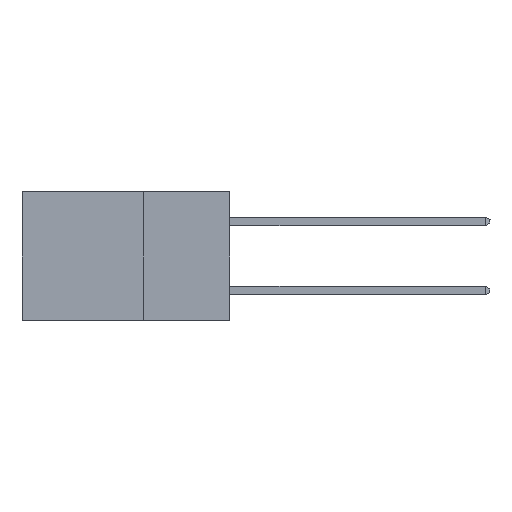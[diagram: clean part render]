
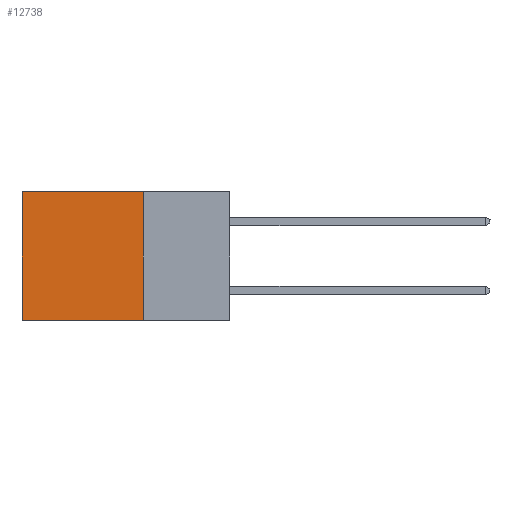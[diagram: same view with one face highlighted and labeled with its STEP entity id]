
A CAD part, left-side view. The second image highlights one B-rep face of the part: STEP entity #12738.
In plain terms, the highlighted planar face has unit normal (-1, 0, 0).
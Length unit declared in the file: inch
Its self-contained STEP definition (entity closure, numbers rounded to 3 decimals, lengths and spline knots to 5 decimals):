
#794 = CARTESIAN_POINT ( 'NONE',  ( 0.2615, 0.25, -0.37 ) ) ;
#1117 = LINE ( 'NONE', #12766, #20195 ) ;
#1715 = DIRECTION ( 'NONE',  ( 0., 0., -1. ) ) ;
#2967 = VECTOR ( 'NONE', #14169, 39.37008 ) ;
#3172 = EDGE_CURVE ( 'NONE', #8773, #21862, #4746, .T. ) ;
#3220 = DIRECTION ( 'NONE',  ( 0., 0., -1. ) ) ;
#3785 = VECTOR ( 'NONE', #20933, 39.37008 ) ;
#4746 = LINE ( 'NONE', #794, #2967 ) ;
#4947 = DIRECTION ( 'NONE',  ( 0., 0., -1. ) ) ;
#7156 = ORIENTED_EDGE ( 'NONE', *, *, #23977, .T. ) ;
#7717 = EDGE_LOOP ( 'NONE', ( #7156, #15749, #22867, #10553 ) ) ;
#8773 = VERTEX_POINT ( 'NONE', #22899 ) ;
#8784 = EDGE_CURVE ( 'NONE', #11501, #8773, #16965, .T. ) ;
#9780 = CARTESIAN_POINT ( 'NONE',  ( 0.2615, 0.25, -0.37 ) ) ;
#10523 = CARTESIAN_POINT ( 'NONE',  ( 0.2615, 0.25, 0. ) ) ;
#10553 = ORIENTED_EDGE ( 'NONE', *, *, #14288, .T. ) ;
#11501 = VERTEX_POINT ( 'NONE', #20447 ) ;
#12738 = ADVANCED_FACE ( 'NONE', ( #16235 ), #18585, .F. ) ;
#12766 = CARTESIAN_POINT ( 'NONE',  ( 0.2615, 0.6, -0.37 ) ) ;
#14169 = DIRECTION ( 'NONE',  ( 0., 1., 0. ) ) ;
#14288 = EDGE_CURVE ( 'NONE', #11501, #18589, #21653, .T. ) ;
#14877 = DIRECTION ( 'NONE',  ( 1., 0., 0. ) ) ;
#15265 = AXIS2_PLACEMENT_3D ( 'NONE', #20294, #14877, #3220 ) ;
#15749 = ORIENTED_EDGE ( 'NONE', *, *, #3172, .F. ) ;
#16235 = FACE_OUTER_BOUND ( 'NONE', #7717, .T. ) ;
#16369 = VECTOR ( 'NONE', #1715, 39.37008 ) ;
#16965 = LINE ( 'NONE', #9780, #16369 ) ;
#18585 = PLANE ( 'NONE',  #15265 ) ;
#18589 = VERTEX_POINT ( 'NONE', #19544 ) ;
#19544 = CARTESIAN_POINT ( 'NONE',  ( 0.2615, 0.6, 0. ) ) ;
#20195 = VECTOR ( 'NONE', #4947, 39.37008 ) ;
#20294 = CARTESIAN_POINT ( 'NONE',  ( 0.2615, 0.25, -0.37 ) ) ;
#20447 = CARTESIAN_POINT ( 'NONE',  ( 0.2615, 0.25, 0. ) ) ;
#20464 = CARTESIAN_POINT ( 'NONE',  ( 0.2615, 0.6, -0.37 ) ) ;
#20933 = DIRECTION ( 'NONE',  ( 0., 1., 0. ) ) ;
#21653 = LINE ( 'NONE', #10523, #3785 ) ;
#21862 = VERTEX_POINT ( 'NONE', #20464 ) ;
#22867 = ORIENTED_EDGE ( 'NONE', *, *, #8784, .F. ) ;
#22899 = CARTESIAN_POINT ( 'NONE',  ( 0.2615, 0.25, -0.37 ) ) ;
#23977 = EDGE_CURVE ( 'NONE', #18589, #21862, #1117, .T. ) ;
